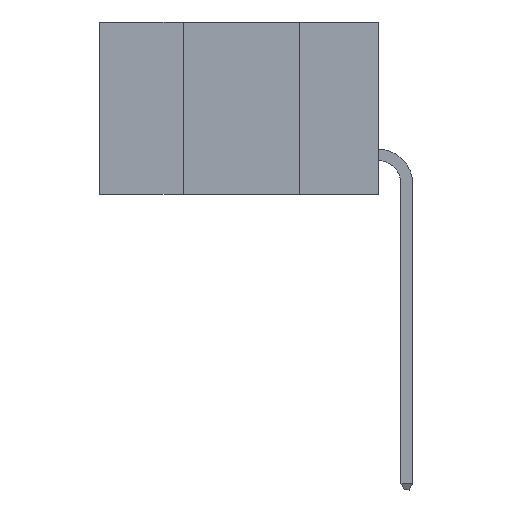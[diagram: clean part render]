
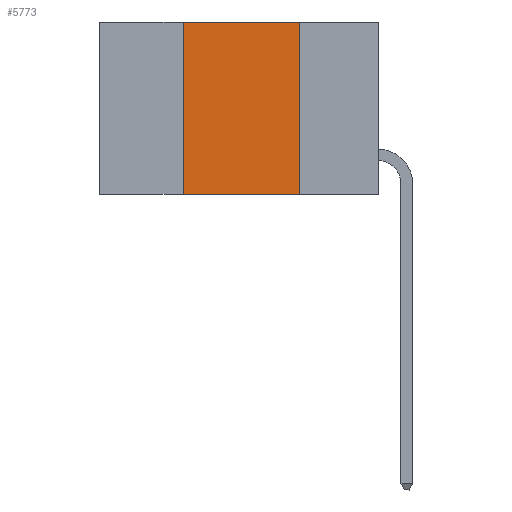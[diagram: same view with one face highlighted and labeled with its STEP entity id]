
A CAD part, left-side view. The second image highlights one B-rep face of the part: STEP entity #5773.
In plain terms, the highlighted planar face has unit normal (-1, 0, 0).
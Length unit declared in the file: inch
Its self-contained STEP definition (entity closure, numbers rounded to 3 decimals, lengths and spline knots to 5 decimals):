
#169 = VERTEX_POINT ( 'NONE', #19645 ) ;
#1332 = CARTESIAN_POINT ( 'NONE',  ( 0., 0.17, 0. ) ) ;
#2742 = CARTESIAN_POINT ( 'NONE',  ( 0., 0.6, -0.37 ) ) ;
#2896 = LINE ( 'NONE', #2742, #22463 ) ;
#3043 = LINE ( 'NONE', #3677, #16085 ) ;
#3230 = ORIENTED_EDGE ( 'NONE', *, *, #16757, .F. ) ;
#3677 = CARTESIAN_POINT ( 'NONE',  ( 0., 0.6, 0. ) ) ;
#3987 = ORIENTED_EDGE ( 'NONE', *, *, #20665, .F. ) ;
#5474 = DIRECTION ( 'NONE',  ( 0., 0., 1. ) ) ;
#5734 = VERTEX_POINT ( 'NONE', #13812 ) ;
#5773 = ADVANCED_FACE ( 'NONE', ( #29200 ), #25250, .F. ) ;
#7906 = VERTEX_POINT ( 'NONE', #11526 ) ;
#8111 = ORIENTED_EDGE ( 'NONE', *, *, #17788, .F. ) ;
#9133 = LINE ( 'NONE', #17767, #28668 ) ;
#11207 = DIRECTION ( 'NONE',  ( 0., -1., 0. ) ) ;
#11526 = CARTESIAN_POINT ( 'NONE',  ( 0., 0.17, -0.37 ) ) ;
#13145 = CARTESIAN_POINT ( 'NONE',  ( 0., 0.6, 0. ) ) ;
#13803 = DIRECTION ( 'NONE',  ( 1., 0., 0. ) ) ;
#13812 = CARTESIAN_POINT ( 'NONE',  ( 0., 0.42, -0.37 ) ) ;
#15300 = VERTEX_POINT ( 'NONE', #25767 ) ;
#15719 = EDGE_CURVE ( 'NONE', #5734, #7906, #2896, .T. ) ;
#16085 = VECTOR ( 'NONE', #11207, 39.37008 ) ;
#16757 = EDGE_CURVE ( 'NONE', #15300, #7906, #22767, .T. ) ;
#17767 = CARTESIAN_POINT ( 'NONE',  ( 0., 0.42, 0. ) ) ;
#17788 = EDGE_CURVE ( 'NONE', #5734, #169, #9133, .T. ) ;
#18955 = ORIENTED_EDGE ( 'NONE', *, *, #15719, .T. ) ;
#19645 = CARTESIAN_POINT ( 'NONE',  ( 0., 0.42, 0. ) ) ;
#19903 = DIRECTION ( 'NONE',  ( 0., -1., 0. ) ) ;
#20665 = EDGE_CURVE ( 'NONE', #169, #15300, #3043, .T. ) ;
#20866 = AXIS2_PLACEMENT_3D ( 'NONE', #13145, #13803, #24898 ) ;
#21019 = DIRECTION ( 'NONE',  ( 0., 0., -1. ) ) ;
#21989 = VECTOR ( 'NONE', #21019, 39.37008 ) ;
#22463 = VECTOR ( 'NONE', #19903, 39.37008 ) ;
#22767 = LINE ( 'NONE', #1332, #21989 ) ;
#24898 = DIRECTION ( 'NONE',  ( 0., 0., -1. ) ) ;
#25250 = PLANE ( 'NONE',  #20866 ) ;
#25767 = CARTESIAN_POINT ( 'NONE',  ( 0., 0.17, 0. ) ) ;
#28668 = VECTOR ( 'NONE', #5474, 39.37008 ) ;
#28736 = EDGE_LOOP ( 'NONE', ( #3230, #3987, #8111, #18955 ) ) ;
#29200 = FACE_OUTER_BOUND ( 'NONE', #28736, .T. ) ;
